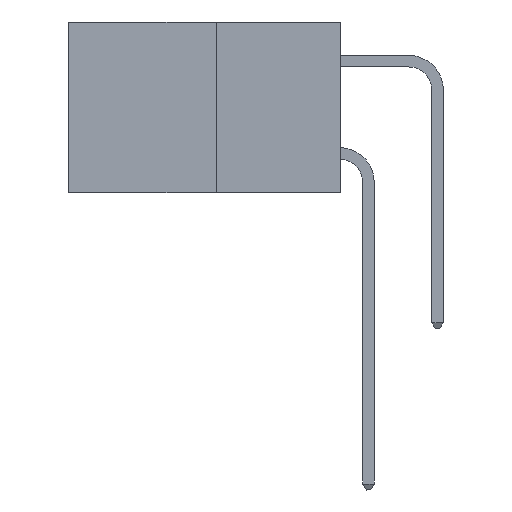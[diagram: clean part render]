
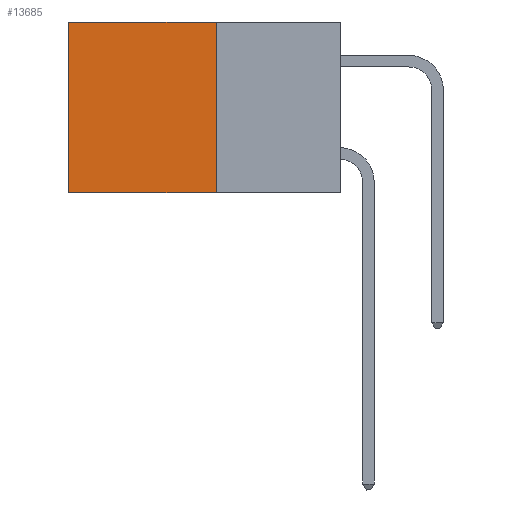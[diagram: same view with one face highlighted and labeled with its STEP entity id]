
A CAD part, left-side view. The second image highlights one B-rep face of the part: STEP entity #13685.
In plain terms, the highlighted planar face has unit normal (-1, 0, 0).
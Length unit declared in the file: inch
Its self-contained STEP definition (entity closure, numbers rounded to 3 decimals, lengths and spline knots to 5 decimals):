
#1937 = LINE ( 'NONE', #13487, #30644 ) ;
#2928 = VECTOR ( 'NONE', #17679, 39.37008 ) ;
#4219 = VERTEX_POINT ( 'NONE', #21543 ) ;
#5134 = EDGE_CURVE ( 'NONE', #29832, #24544, #27281, .T. ) ;
#5498 = VECTOR ( 'NONE', #6992, 39.37008 ) ;
#6621 = ORIENTED_EDGE ( 'NONE', *, *, #32646, .F. ) ;
#6992 = DIRECTION ( 'NONE',  ( 0., 0., -1. ) ) ;
#9918 = CARTESIAN_POINT ( 'NONE',  ( 0.277, 0.59, 0. ) ) ;
#10369 = CARTESIAN_POINT ( 'NONE',  ( 0.277, 0.59, -0.37 ) ) ;
#11680 = VERTEX_POINT ( 'NONE', #10369 ) ;
#12284 = ORIENTED_EDGE ( 'NONE', *, *, #16981, .F. ) ;
#13487 = CARTESIAN_POINT ( 'NONE',  ( 0.277, 0.27, -0.37 ) ) ;
#13685 = ADVANCED_FACE ( 'NONE', ( #15947 ), #29356, .F. ) ;
#14737 = ORIENTED_EDGE ( 'NONE', *, *, #5134, .T. ) ;
#15070 = CARTESIAN_POINT ( 'NONE',  ( 0.277, 0.27, -0.37 ) ) ;
#15947 = FACE_OUTER_BOUND ( 'NONE', #31707, .T. ) ;
#16108 = DIRECTION ( 'NONE',  ( 0., 0., -1. ) ) ;
#16981 = EDGE_CURVE ( 'NONE', #29832, #4219, #24445, .T. ) ;
#17679 = DIRECTION ( 'NONE',  ( 0., 0., -1. ) ) ;
#18141 = ORIENTED_EDGE ( 'NONE', *, *, #24442, .T. ) ;
#21347 = AXIS2_PLACEMENT_3D ( 'NONE', #23987, #32109, #16108 ) ;
#21543 = CARTESIAN_POINT ( 'NONE',  ( 0.277, 0.27, -0.37 ) ) ;
#23097 = CARTESIAN_POINT ( 'NONE',  ( 0.277, 0.59, -0.37 ) ) ;
#23623 = DIRECTION ( 'NONE',  ( 0., 1., 0. ) ) ;
#23987 = CARTESIAN_POINT ( 'NONE',  ( 0.277, 0.27, -0.37 ) ) ;
#24442 = EDGE_CURVE ( 'NONE', #24544, #11680, #33236, .T. ) ;
#24445 = LINE ( 'NONE', #15070, #2928 ) ;
#24544 = VERTEX_POINT ( 'NONE', #9918 ) ;
#26436 = VECTOR ( 'NONE', #23623, 39.37008 ) ;
#27281 = LINE ( 'NONE', #29340, #26436 ) ;
#27379 = CARTESIAN_POINT ( 'NONE',  ( 0.277, 0.27, 0. ) ) ;
#29340 = CARTESIAN_POINT ( 'NONE',  ( 0.277, 0.27, 0. ) ) ;
#29356 = PLANE ( 'NONE',  #21347 ) ;
#29389 = DIRECTION ( 'NONE',  ( 0., 1., 0. ) ) ;
#29832 = VERTEX_POINT ( 'NONE', #27379 ) ;
#30644 = VECTOR ( 'NONE', #29389, 39.37008 ) ;
#31707 = EDGE_LOOP ( 'NONE', ( #18141, #6621, #12284, #14737 ) ) ;
#32109 = DIRECTION ( 'NONE',  ( 1., 0., 0. ) ) ;
#32646 = EDGE_CURVE ( 'NONE', #4219, #11680, #1937, .T. ) ;
#33236 = LINE ( 'NONE', #23097, #5498 ) ;
